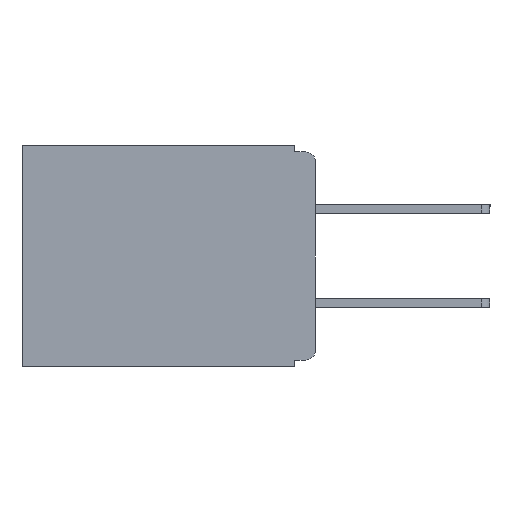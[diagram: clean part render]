
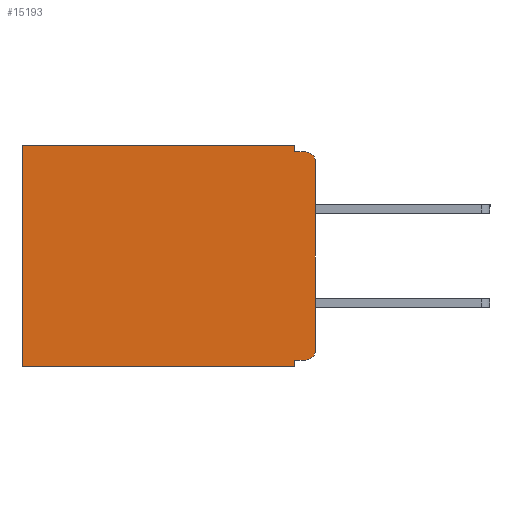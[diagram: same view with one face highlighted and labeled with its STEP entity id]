
A CAD part, left-side view. The second image highlights one B-rep face of the part: STEP entity #15193.
In plain terms, the highlighted planar face has unit normal (-1, 0, 0).
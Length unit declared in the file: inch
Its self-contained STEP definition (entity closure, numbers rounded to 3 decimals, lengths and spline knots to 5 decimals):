
#397 = CARTESIAN_POINT ( 'NONE',  ( 0.3, 0.437, 0. ) ) ;
#460 = LINE ( 'NONE', #24367, #1788 ) ;
#534 = LINE ( 'NONE', #9968, #21889 ) ;
#1515 = VERTEX_POINT ( 'NONE', #11944 ) ;
#1788 = VECTOR ( 'NONE', #12730, 39.37008 ) ;
#2095 = LINE ( 'NONE', #14000, #12285 ) ;
#2647 = EDGE_CURVE ( 'NONE', #7103, #15429, #9083, .T. ) ;
#2845 = DIRECTION ( 'NONE',  ( 0., 0., -1. ) ) ;
#3273 = VECTOR ( 'NONE', #6584, 39.37008 ) ;
#3472 = PLANE ( 'NONE',  #21174 ) ;
#3871 = ORIENTED_EDGE ( 'NONE', *, *, #11175, .T. ) ;
#3943 = DIRECTION ( 'NONE',  ( 0., 0., -1. ) ) ;
#3978 = LINE ( 'NONE', #6921, #14066 ) ;
#4712 = EDGE_CURVE ( 'NONE', #16114, #9640, #8682, .T. ) ;
#5191 = EDGE_CURVE ( 'NONE', #25283, #9640, #8022, .T. ) ;
#5305 = DIRECTION ( 'NONE',  ( -1., 0., 0. ) ) ;
#5550 = CARTESIAN_POINT ( 'NONE',  ( 0.3, 0.031, -0.33 ) ) ;
#6119 = VERTEX_POINT ( 'NONE', #397 ) ;
#6584 = DIRECTION ( 'NONE',  ( 0., 0., -1. ) ) ;
#6771 = ORIENTED_EDGE ( 'NONE', *, *, #9272, .T. ) ;
#6921 = CARTESIAN_POINT ( 'NONE',  ( 0.3, 0., 0. ) ) ;
#7103 = VERTEX_POINT ( 'NONE', #22565 ) ;
#7560 = DIRECTION ( 'NONE',  ( 0., 0., -1. ) ) ;
#8022 = CIRCLE ( 'NONE', #13270, 0.015 ) ;
#8237 = CARTESIAN_POINT ( 'NONE',  ( 0.3, 0., -0.025 ) ) ;
#8682 = LINE ( 'NONE', #10858, #3273 ) ;
#9083 = LINE ( 'NONE', #16882, #24710 ) ;
#9272 = EDGE_CURVE ( 'NONE', #6119, #1515, #460, .T. ) ;
#9640 = VERTEX_POINT ( 'NONE', #9862 ) ;
#9862 = CARTESIAN_POINT ( 'NONE',  ( 0.3, 0., -0.305 ) ) ;
#9968 = CARTESIAN_POINT ( 'NONE',  ( 0.3, 0., -0.32 ) ) ;
#10053 = CARTESIAN_POINT ( 'NONE',  ( 0.3, 0., -0.01 ) ) ;
#10652 = EDGE_CURVE ( 'NONE', #16114, #19359, #11288, .T. ) ;
#10858 = CARTESIAN_POINT ( 'NONE',  ( 0.3, 0., -0.33 ) ) ;
#11175 = EDGE_CURVE ( 'NONE', #7103, #6119, #3978, .T. ) ;
#11288 = CIRCLE ( 'NONE', #16386, 0.015 ) ;
#11593 = ORIENTED_EDGE ( 'NONE', *, *, #2647, .F. ) ;
#11944 = CARTESIAN_POINT ( 'NONE',  ( 0.3, 0.437, -0.33 ) ) ;
#12085 = ORIENTED_EDGE ( 'NONE', *, *, #16019, .F. ) ;
#12285 = VECTOR ( 'NONE', #3943, 39.37008 ) ;
#12730 = DIRECTION ( 'NONE',  ( 0., 0., -1. ) ) ;
#12926 = ORIENTED_EDGE ( 'NONE', *, *, #10652, .T. ) ;
#13175 = ORIENTED_EDGE ( 'NONE', *, *, #4712, .F. ) ;
#13270 = AXIS2_PLACEMENT_3D ( 'NONE', #16213, #16167, #16160 ) ;
#13392 = VECTOR ( 'NONE', #23772, 39.37008 ) ;
#14000 = CARTESIAN_POINT ( 'NONE',  ( 0.3, 0.031, -0.33 ) ) ;
#14066 = VECTOR ( 'NONE', #14978, 39.37008 ) ;
#14814 = EDGE_CURVE ( 'NONE', #20642, #1515, #17194, .T. ) ;
#14978 = DIRECTION ( 'NONE',  ( 0., 1., 0. ) ) ;
#15193 = ADVANCED_FACE ( 'NONE', ( #22253 ), #3472, .F. ) ;
#15403 = ORIENTED_EDGE ( 'NONE', *, *, #25605, .F. ) ;
#15429 = VERTEX_POINT ( 'NONE', #20107 ) ;
#16019 = EDGE_CURVE ( 'NONE', #25283, #23869, #534, .T. ) ;
#16114 = VERTEX_POINT ( 'NONE', #8237 ) ;
#16160 = DIRECTION ( 'NONE',  ( 0., 0., -1. ) ) ;
#16167 = DIRECTION ( 'NONE',  ( -1., 0., 0. ) ) ;
#16213 = CARTESIAN_POINT ( 'NONE',  ( 0.3, 0.015, -0.305 ) ) ;
#16386 = AXIS2_PLACEMENT_3D ( 'NONE', #17398, #5305, #19352 ) ;
#16882 = CARTESIAN_POINT ( 'NONE',  ( 0.3, 0.031, 0. ) ) ;
#17134 = ORIENTED_EDGE ( 'NONE', *, *, #14814, .F. ) ;
#17194 = LINE ( 'NONE', #18309, #24896 ) ;
#17245 = ORIENTED_EDGE ( 'NONE', *, *, #22488, .F. ) ;
#17398 = CARTESIAN_POINT ( 'NONE',  ( 0.3, 0.015, -0.025 ) ) ;
#17588 = CARTESIAN_POINT ( 'NONE',  ( 0.3, 0., -0.33 ) ) ;
#18156 = CARTESIAN_POINT ( 'NONE',  ( 0.3, 0.015, -0.32 ) ) ;
#18309 = CARTESIAN_POINT ( 'NONE',  ( 0.3, 0., -0.33 ) ) ;
#19317 = CARTESIAN_POINT ( 'NONE',  ( 0.3, 0.031, -0.32 ) ) ;
#19352 = DIRECTION ( 'NONE',  ( 0., 0., -1. ) ) ;
#19359 = VERTEX_POINT ( 'NONE', #24281 ) ;
#19531 = DIRECTION ( 'NONE',  ( 1., 0., 0. ) ) ;
#19662 = EDGE_LOOP ( 'NONE', ( #13175, #12926, #17245, #11593, #3871, #6771, #17134, #15403, #12085, #20844 ) ) ;
#20107 = CARTESIAN_POINT ( 'NONE',  ( 0.3, 0.031, -0.01 ) ) ;
#20214 = DIRECTION ( 'NONE',  ( 0., 1., 0. ) ) ;
#20642 = VERTEX_POINT ( 'NONE', #5550 ) ;
#20844 = ORIENTED_EDGE ( 'NONE', *, *, #5191, .T. ) ;
#21174 = AXIS2_PLACEMENT_3D ( 'NONE', #17588, #19531, #7560 ) ;
#21889 = VECTOR ( 'NONE', #23688, 39.37008 ) ;
#22253 = FACE_OUTER_BOUND ( 'NONE', #19662, .T. ) ;
#22488 = EDGE_CURVE ( 'NONE', #15429, #19359, #22564, .T. ) ;
#22564 = LINE ( 'NONE', #10053, #13392 ) ;
#22565 = CARTESIAN_POINT ( 'NONE',  ( 0.3, 0.031, 0. ) ) ;
#23688 = DIRECTION ( 'NONE',  ( 0., 1., 0. ) ) ;
#23772 = DIRECTION ( 'NONE',  ( 0., -1., 0. ) ) ;
#23869 = VERTEX_POINT ( 'NONE', #19317 ) ;
#24281 = CARTESIAN_POINT ( 'NONE',  ( 0.3, 0.015, -0.01 ) ) ;
#24367 = CARTESIAN_POINT ( 'NONE',  ( 0.3, 0.437, -0.33 ) ) ;
#24710 = VECTOR ( 'NONE', #2845, 39.37008 ) ;
#24896 = VECTOR ( 'NONE', #20214, 39.37008 ) ;
#25283 = VERTEX_POINT ( 'NONE', #18156 ) ;
#25605 = EDGE_CURVE ( 'NONE', #23869, #20642, #2095, .T. ) ;
